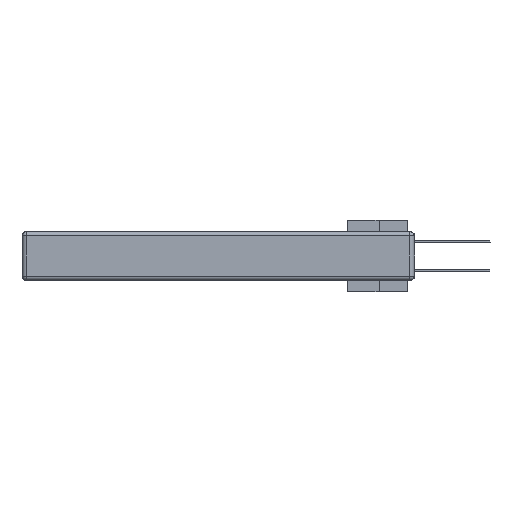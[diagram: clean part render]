
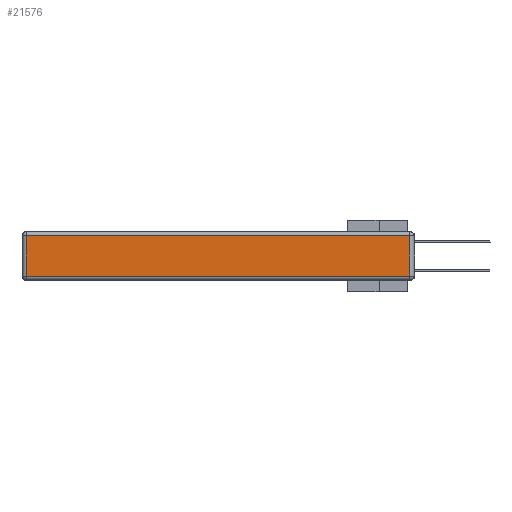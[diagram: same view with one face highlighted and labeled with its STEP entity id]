
A CAD part, left-side view. The second image highlights one B-rep face of the part: STEP entity #21576.
In plain terms, the highlighted planar face has unit normal (-1, 0, 0).
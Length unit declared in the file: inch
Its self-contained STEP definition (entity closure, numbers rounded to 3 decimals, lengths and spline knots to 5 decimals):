
#243 = VECTOR ( 'NONE', #1903, 39.37008 ) ;
#1562 = DIRECTION ( 'NONE',  ( 0., -1., 0. ) ) ;
#1903 = DIRECTION ( 'NONE',  ( 0., 0., 1. ) ) ;
#2176 = FACE_OUTER_BOUND ( 'NONE', #20350, .T. ) ;
#3700 = DIRECTION ( 'NONE',  ( 0., 1., 0. ) ) ;
#4003 = CARTESIAN_POINT ( 'NONE',  ( 0., 0.03, -0.343 ) ) ;
#4497 = LINE ( 'NONE', #17214, #21820 ) ;
#4795 = LINE ( 'NONE', #23183, #19630 ) ;
#5006 = EDGE_CURVE ( 'NONE', #25012, #28936, #4795, .T. ) ;
#6302 = ORIENTED_EDGE ( 'NONE', *, *, #18909, .T. ) ;
#6374 = CARTESIAN_POINT ( 'NONE',  ( 0., 0.03, -0.03 ) ) ;
#6635 = VERTEX_POINT ( 'NONE', #6374 ) ;
#7554 = DIRECTION ( 'NONE',  ( 0., 0., -1. ) ) ;
#7711 = LINE ( 'NONE', #4003, #243 ) ;
#8441 = EDGE_CURVE ( 'NONE', #17024, #6635, #7711, .T. ) ;
#11319 = AXIS2_PLACEMENT_3D ( 'NONE', #12759, #28591, #15026 ) ;
#12759 = CARTESIAN_POINT ( 'NONE',  ( 0., 0., -0.343 ) ) ;
#13156 = CARTESIAN_POINT ( 'NONE',  ( 0., 0., -0.313 ) ) ;
#13259 = CARTESIAN_POINT ( 'NONE',  ( 0., 2.72, -0.313 ) ) ;
#15026 = DIRECTION ( 'NONE',  ( 0., 0., 1. ) ) ;
#15838 = ORIENTED_EDGE ( 'NONE', *, *, #5006, .T. ) ;
#16668 = CARTESIAN_POINT ( 'NONE',  ( 0., 2.72, -0.03 ) ) ;
#17024 = VERTEX_POINT ( 'NONE', #19351 ) ;
#17214 = CARTESIAN_POINT ( 'NONE',  ( 0., 2.75, -0.03 ) ) ;
#17234 = VECTOR ( 'NONE', #1562, 39.37008 ) ;
#18909 = EDGE_CURVE ( 'NONE', #6635, #25012, #4497, .T. ) ;
#19351 = CARTESIAN_POINT ( 'NONE',  ( 0., 0.03, -0.313 ) ) ;
#19630 = VECTOR ( 'NONE', #7554, 39.37008 ) ;
#20350 = EDGE_LOOP ( 'NONE', ( #21243, #21649, #6302, #15838 ) ) ;
#21243 = ORIENTED_EDGE ( 'NONE', *, *, #23804, .T. ) ;
#21576 = ADVANCED_FACE ( 'NONE', ( #2176 ), #22226, .T. ) ;
#21649 = ORIENTED_EDGE ( 'NONE', *, *, #8441, .T. ) ;
#21820 = VECTOR ( 'NONE', #3700, 39.37008 ) ;
#22226 = PLANE ( 'NONE',  #11319 ) ;
#23183 = CARTESIAN_POINT ( 'NONE',  ( 0., 2.72, -0.343 ) ) ;
#23804 = EDGE_CURVE ( 'NONE', #28936, #17024, #29310, .T. ) ;
#25012 = VERTEX_POINT ( 'NONE', #16668 ) ;
#28591 = DIRECTION ( 'NONE',  ( -1., 0., 0. ) ) ;
#28936 = VERTEX_POINT ( 'NONE', #13259 ) ;
#29310 = LINE ( 'NONE', #13156, #17234 ) ;
